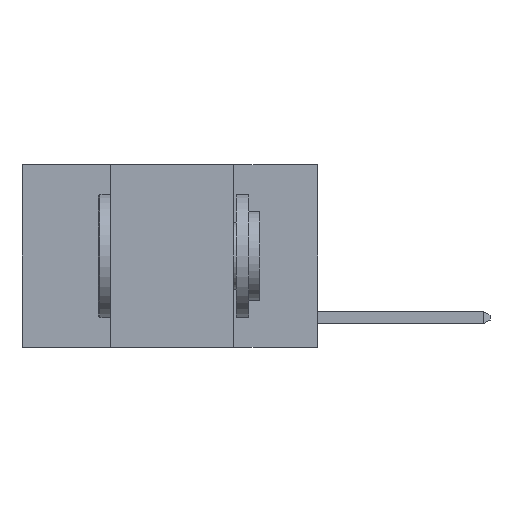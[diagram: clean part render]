
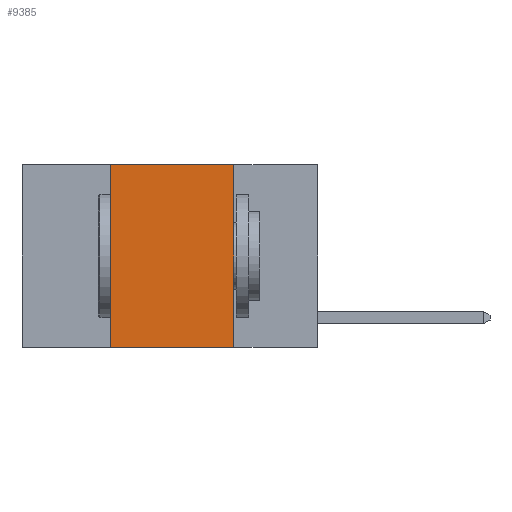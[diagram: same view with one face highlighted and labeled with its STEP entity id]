
A CAD part, left-side view. The second image highlights one B-rep face of the part: STEP entity #9385.
In plain terms, the highlighted planar face has unit normal (-1, 0, 0).
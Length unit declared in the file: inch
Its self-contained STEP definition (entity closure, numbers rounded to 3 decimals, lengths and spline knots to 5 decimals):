
#51 = DIRECTION ( 'NONE',  ( 0., 0., -1. ) ) ;
#1048 = CARTESIAN_POINT ( 'NONE',  ( 0., 0.17, 0. ) ) ;
#1392 = CARTESIAN_POINT ( 'NONE',  ( 0., 0.42, 0. ) ) ;
#1462 = CARTESIAN_POINT ( 'NONE',  ( 0., 0.42, -0.37 ) ) ;
#1713 = CARTESIAN_POINT ( 'NONE',  ( 0., 0.17, -0.37 ) ) ;
#2013 = EDGE_CURVE ( 'NONE', #4281, #2741, #5977, .T. ) ;
#2076 = LINE ( 'NONE', #4225, #4321 ) ;
#2741 = VERTEX_POINT ( 'NONE', #1048 ) ;
#2844 = FACE_OUTER_BOUND ( 'NONE', #8880, .T. ) ;
#3213 = DIRECTION ( 'NONE',  ( 0., 0., 1. ) ) ;
#3334 = DIRECTION ( 'NONE',  ( 0., -1., 0. ) ) ;
#3573 = PLANE ( 'NONE',  #4019 ) ;
#3856 = VERTEX_POINT ( 'NONE', #1713 ) ;
#4019 = AXIS2_PLACEMENT_3D ( 'NONE', #4390, #5291, #51 ) ;
#4225 = CARTESIAN_POINT ( 'NONE',  ( 0., 0.17, 0. ) ) ;
#4281 = VERTEX_POINT ( 'NONE', #1392 ) ;
#4321 = VECTOR ( 'NONE', #7557, 39.37008 ) ;
#4390 = CARTESIAN_POINT ( 'NONE',  ( 0., 0.6, 0. ) ) ;
#4877 = ORIENTED_EDGE ( 'NONE', *, *, #8613, .F. ) ;
#5145 = ORIENTED_EDGE ( 'NONE', *, *, #8105, .F. ) ;
#5291 = DIRECTION ( 'NONE',  ( 1., 0., 0. ) ) ;
#5676 = LINE ( 'NONE', #10693, #7621 ) ;
#5977 = LINE ( 'NONE', #8235, #10513 ) ;
#6586 = LINE ( 'NONE', #8208, #8713 ) ;
#7113 = ORIENTED_EDGE ( 'NONE', *, *, #2013, .F. ) ;
#7368 = ORIENTED_EDGE ( 'NONE', *, *, #7568, .T. ) ;
#7557 = DIRECTION ( 'NONE',  ( 0., 0., -1. ) ) ;
#7568 = EDGE_CURVE ( 'NONE', #8139, #3856, #5676, .T. ) ;
#7621 = VECTOR ( 'NONE', #3334, 39.37008 ) ;
#8105 = EDGE_CURVE ( 'NONE', #8139, #4281, #6586, .T. ) ;
#8139 = VERTEX_POINT ( 'NONE', #1462 ) ;
#8208 = CARTESIAN_POINT ( 'NONE',  ( 0., 0.42, 0. ) ) ;
#8223 = DIRECTION ( 'NONE',  ( 0., -1., 0. ) ) ;
#8235 = CARTESIAN_POINT ( 'NONE',  ( 0., 0.6, 0. ) ) ;
#8613 = EDGE_CURVE ( 'NONE', #2741, #3856, #2076, .T. ) ;
#8713 = VECTOR ( 'NONE', #3213, 39.37008 ) ;
#8880 = EDGE_LOOP ( 'NONE', ( #4877, #7113, #5145, #7368 ) ) ;
#9385 = ADVANCED_FACE ( 'NONE', ( #2844 ), #3573, .F. ) ;
#10513 = VECTOR ( 'NONE', #8223, 39.37008 ) ;
#10693 = CARTESIAN_POINT ( 'NONE',  ( 0., 0.6, -0.37 ) ) ;
